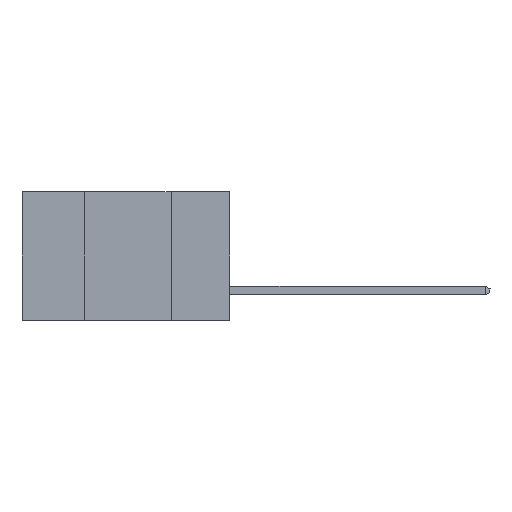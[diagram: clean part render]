
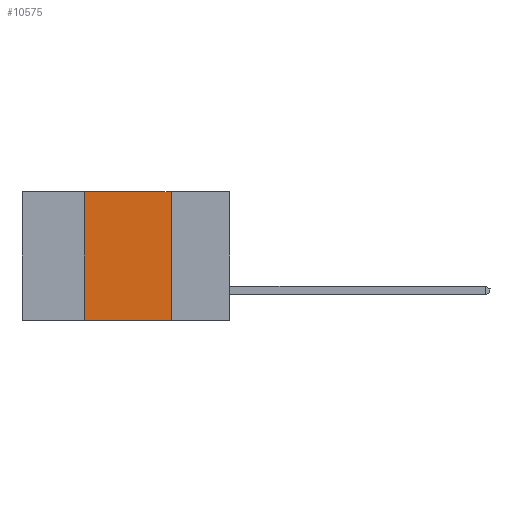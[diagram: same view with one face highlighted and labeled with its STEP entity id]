
A CAD part, left-side view. The second image highlights one B-rep face of the part: STEP entity #10575.
In plain terms, the highlighted planar face has unit normal (-1, 0, 0).
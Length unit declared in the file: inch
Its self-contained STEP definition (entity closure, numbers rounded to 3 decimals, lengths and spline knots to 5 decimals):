
#121 = DIRECTION ( 'NONE',  ( 0., -1., 0. ) ) ;
#148 = VECTOR ( 'NONE', #8220, 39.37008 ) ;
#502 = VERTEX_POINT ( 'NONE', #2357 ) ;
#823 = CARTESIAN_POINT ( 'NONE',  ( 0., 0.42, -0.37 ) ) ;
#844 = VECTOR ( 'NONE', #9528, 39.37008 ) ;
#981 = EDGE_LOOP ( 'NONE', ( #5139, #7594, #10560, #10244 ) ) ;
#1660 = VERTEX_POINT ( 'NONE', #8021 ) ;
#2350 = LINE ( 'NONE', #9684, #148 ) ;
#2355 = PLANE ( 'NONE',  #9533 ) ;
#2357 = CARTESIAN_POINT ( 'NONE',  ( 0., 0.17, 0. ) ) ;
#2546 = LINE ( 'NONE', #7589, #9834 ) ;
#3970 = CARTESIAN_POINT ( 'NONE',  ( 0., 0.6, 0. ) ) ;
#4081 = LINE ( 'NONE', #3970, #9780 ) ;
#4366 = EDGE_CURVE ( 'NONE', #1660, #502, #4081, .T. ) ;
#5139 = ORIENTED_EDGE ( 'NONE', *, *, #7569, .F. ) ;
#5449 = DIRECTION ( 'NONE',  ( 1., 0., 0. ) ) ;
#5634 = DIRECTION ( 'NONE',  ( 0., -1., 0. ) ) ;
#6848 = CARTESIAN_POINT ( 'NONE',  ( 0., 0.17, -0.37 ) ) ;
#6931 = VERTEX_POINT ( 'NONE', #823 ) ;
#7299 = CARTESIAN_POINT ( 'NONE',  ( 0., 0.6, 0. ) ) ;
#7569 = EDGE_CURVE ( 'NONE', #502, #7875, #9580, .T. ) ;
#7589 = CARTESIAN_POINT ( 'NONE',  ( 0., 0.6, -0.37 ) ) ;
#7594 = ORIENTED_EDGE ( 'NONE', *, *, #4366, .F. ) ;
#7687 = EDGE_CURVE ( 'NONE', #6931, #1660, #2350, .T. ) ;
#7875 = VERTEX_POINT ( 'NONE', #6848 ) ;
#8015 = FACE_OUTER_BOUND ( 'NONE', #981, .T. ) ;
#8021 = CARTESIAN_POINT ( 'NONE',  ( 0., 0.42, 0. ) ) ;
#8220 = DIRECTION ( 'NONE',  ( 0., 0., 1. ) ) ;
#8559 = EDGE_CURVE ( 'NONE', #6931, #7875, #2546, .T. ) ;
#8713 = CARTESIAN_POINT ( 'NONE',  ( 0., 0.17, -0.37 ) ) ;
#8771 = DIRECTION ( 'NONE',  ( 0., 0., -1. ) ) ;
#9528 = DIRECTION ( 'NONE',  ( 0., 0., -1. ) ) ;
#9533 = AXIS2_PLACEMENT_3D ( 'NONE', #7299, #5449, #8771 ) ;
#9580 = LINE ( 'NONE', #8713, #844 ) ;
#9684 = CARTESIAN_POINT ( 'NONE',  ( 0., 0.42, -0.37 ) ) ;
#9780 = VECTOR ( 'NONE', #5634, 39.37008 ) ;
#9834 = VECTOR ( 'NONE', #121, 39.37008 ) ;
#10244 = ORIENTED_EDGE ( 'NONE', *, *, #8559, .T. ) ;
#10560 = ORIENTED_EDGE ( 'NONE', *, *, #7687, .F. ) ;
#10575 = ADVANCED_FACE ( 'NONE', ( #8015 ), #2355, .F. ) ;
